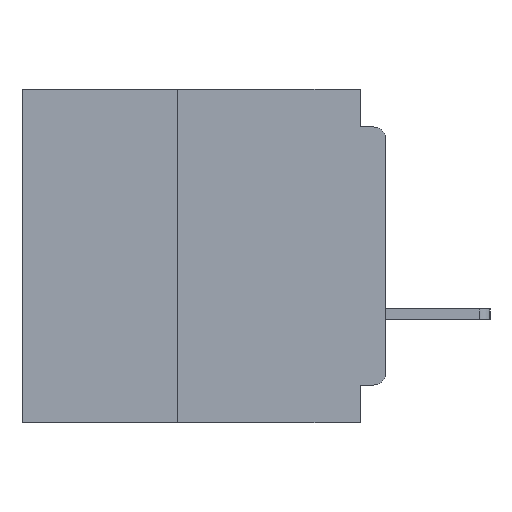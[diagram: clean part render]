
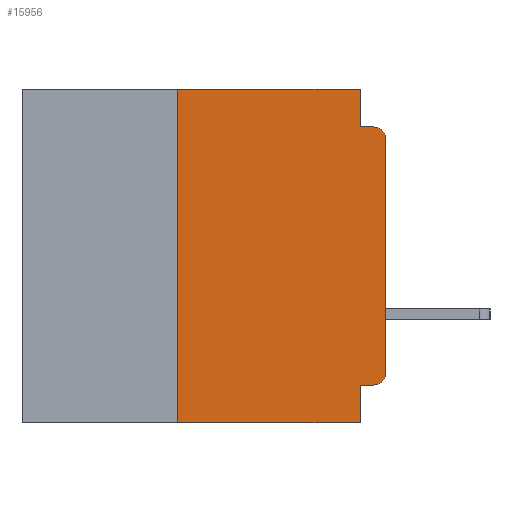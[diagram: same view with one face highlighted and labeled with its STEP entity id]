
A CAD part, left-side view. The second image highlights one B-rep face of the part: STEP entity #15956.
In plain terms, the highlighted planar face has unit normal (-1, 0, 0).
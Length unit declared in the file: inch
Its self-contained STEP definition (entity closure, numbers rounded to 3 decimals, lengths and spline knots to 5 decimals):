
#1579 = CARTESIAN_POINT ( 'NONE',  ( 0., 0.437, -0.4 ) ) ;
#1644 = DIRECTION ( 'NONE',  ( 0., 0., -1. ) ) ;
#3297 = VERTEX_POINT ( 'NONE', #16505 ) ;
#3374 = DIRECTION ( 'NONE',  ( -1., 0., 0. ) ) ;
#5253 = EDGE_CURVE ( 'NONE', #7783, #30090, #43500, .T. ) ;
#5803 = VERTEX_POINT ( 'NONE', #9554 ) ;
#6640 = DIRECTION ( 'NONE',  ( 0., 0., 1. ) ) ;
#7783 = VERTEX_POINT ( 'NONE', #48937 ) ;
#8978 = VERTEX_POINT ( 'NONE', #28548 ) ;
#9554 = CARTESIAN_POINT ( 'NONE',  ( 0., 0.031, -0.4 ) ) ;
#9669 = VECTOR ( 'NONE', #21164, 39.37008 ) ;
#9750 = CARTESIAN_POINT ( 'NONE',  ( 0., 0.015, -0.34 ) ) ;
#10940 = CARTESIAN_POINT ( 'NONE',  ( 0., 0.25, -0.4 ) ) ;
#11114 = LINE ( 'NONE', #27116, #21167 ) ;
#12034 = CARTESIAN_POINT ( 'NONE',  ( 0., 0., 0. ) ) ;
#12304 = VECTOR ( 'NONE', #52144, 39.37008 ) ;
#12464 = ORIENTED_EDGE ( 'NONE', *, *, #52574, .F. ) ;
#12562 = CARTESIAN_POINT ( 'NONE',  ( 0., 0., -0.355 ) ) ;
#12618 = CARTESIAN_POINT ( 'NONE',  ( 0., 0.25, -0.4 ) ) ;
#13251 = EDGE_CURVE ( 'NONE', #3297, #23100, #19534, .T. ) ;
#14091 = DIRECTION ( 'NONE',  ( 0., 0., -1. ) ) ;
#14128 = VECTOR ( 'NONE', #29550, 39.37008 ) ;
#15361 = ORIENTED_EDGE ( 'NONE', *, *, #41898, .T. ) ;
#15956 = ADVANCED_FACE ( 'NONE', ( #37205 ), #22993, .F. ) ;
#15974 = DIRECTION ( 'NONE',  ( 0., 0., 1. ) ) ;
#16505 = CARTESIAN_POINT ( 'NONE',  ( 0., 0.25, 0. ) ) ;
#16544 = ORIENTED_EDGE ( 'NONE', *, *, #5253, .F. ) ;
#16617 = VERTEX_POINT ( 'NONE', #44299 ) ;
#18028 = EDGE_CURVE ( 'NONE', #16617, #44447, #32406, .T. ) ;
#18341 = ORIENTED_EDGE ( 'NONE', *, *, #38912, .T. ) ;
#19534 = LINE ( 'NONE', #46771, #42001 ) ;
#20184 = CARTESIAN_POINT ( 'NONE',  ( 0., 0.015, -0.045 ) ) ;
#20460 = ORIENTED_EDGE ( 'NONE', *, *, #18028, .T. ) ;
#21164 = DIRECTION ( 'NONE',  ( 0., 1., 0. ) ) ;
#21167 = VECTOR ( 'NONE', #31429, 39.37008 ) ;
#22165 = EDGE_CURVE ( 'NONE', #23100, #8978, #11114, .T. ) ;
#22993 = PLANE ( 'NONE',  #26271 ) ;
#23100 = VERTEX_POINT ( 'NONE', #36058 ) ;
#23667 = LINE ( 'NONE', #39546, #12304 ) ;
#25241 = CARTESIAN_POINT ( 'NONE',  ( 0., 0., -0.045 ) ) ;
#25264 = ORIENTED_EDGE ( 'NONE', *, *, #22165, .F. ) ;
#25638 = CIRCLE ( 'NONE', #49632, 0.015 ) ;
#25844 = DIRECTION ( 'NONE',  ( 0., -1., 0. ) ) ;
#26271 = AXIS2_PLACEMENT_3D ( 'NONE', #52357, #27292, #1644 ) ;
#26833 = ORIENTED_EDGE ( 'NONE', *, *, #13251, .F. ) ;
#27116 = CARTESIAN_POINT ( 'NONE',  ( 0., 0.031, 0. ) ) ;
#27292 = DIRECTION ( 'NONE',  ( 1., 0., 0. ) ) ;
#28365 = CARTESIAN_POINT ( 'NONE',  ( 0., 0.031, -0.355 ) ) ;
#28548 = CARTESIAN_POINT ( 'NONE',  ( 0., 0.031, -0.045 ) ) ;
#29007 = CARTESIAN_POINT ( 'NONE',  ( 0., 0.015, -0.06 ) ) ;
#29541 = LINE ( 'NONE', #25241, #14128 ) ;
#29550 = DIRECTION ( 'NONE',  ( 0., -1., 0. ) ) ;
#30090 = VERTEX_POINT ( 'NONE', #28365 ) ;
#31429 = DIRECTION ( 'NONE',  ( 0., 0., -1. ) ) ;
#32406 = CIRCLE ( 'NONE', #41478, 0.015 ) ;
#33193 = ORIENTED_EDGE ( 'NONE', *, *, #40878, .T. ) ;
#33266 = DIRECTION ( 'NONE',  ( 0., 0., -1. ) ) ;
#33924 = VECTOR ( 'NONE', #35680, 39.37008 ) ;
#34425 = EDGE_CURVE ( 'NONE', #8978, #44447, #29541, .T. ) ;
#35285 = EDGE_LOOP ( 'NONE', ( #33193, #20460, #38125, #25264, #26833, #12464, #15361, #45844, #16544, #18341 ) ) ;
#35515 = VERTEX_POINT ( 'NONE', #12618 ) ;
#35680 = DIRECTION ( 'NONE',  ( 0., -1., 0. ) ) ;
#36058 = CARTESIAN_POINT ( 'NONE',  ( 0., 0.031, 0. ) ) ;
#37205 = FACE_OUTER_BOUND ( 'NONE', #35285, .T. ) ;
#38125 = ORIENTED_EDGE ( 'NONE', *, *, #34425, .F. ) ;
#38912 = EDGE_CURVE ( 'NONE', #7783, #54745, #25638, .T. ) ;
#39437 = DIRECTION ( 'NONE',  ( -1., 0., 0. ) ) ;
#39546 = CARTESIAN_POINT ( 'NONE',  ( 0., 0.031, -0.4 ) ) ;
#40878 = EDGE_CURVE ( 'NONE', #54745, #16617, #54219, .T. ) ;
#41478 = AXIS2_PLACEMENT_3D ( 'NONE', #29007, #3374, #33266 ) ;
#41573 = VECTOR ( 'NONE', #6640, 39.37008 ) ;
#41898 = EDGE_CURVE ( 'NONE', #35515, #5803, #45000, .T. ) ;
#42001 = VECTOR ( 'NONE', #25844, 39.37008 ) ;
#43500 = LINE ( 'NONE', #12562, #9669 ) ;
#44299 = CARTESIAN_POINT ( 'NONE',  ( 0., 0., -0.06 ) ) ;
#44447 = VERTEX_POINT ( 'NONE', #20184 ) ;
#44469 = VECTOR ( 'NONE', #15974, 39.37008 ) ;
#45000 = LINE ( 'NONE', #1579, #33924 ) ;
#45844 = ORIENTED_EDGE ( 'NONE', *, *, #53527, .F. ) ;
#46771 = CARTESIAN_POINT ( 'NONE',  ( 0., 0.437, 0. ) ) ;
#48225 = CARTESIAN_POINT ( 'NONE',  ( 0., 0., -0.34 ) ) ;
#48937 = CARTESIAN_POINT ( 'NONE',  ( 0., 0.015, -0.355 ) ) ;
#49632 = AXIS2_PLACEMENT_3D ( 'NONE', #9750, #39437, #14091 ) ;
#52144 = DIRECTION ( 'NONE',  ( 0., 0., -1. ) ) ;
#52357 = CARTESIAN_POINT ( 'NONE',  ( 0., 0.437, 0. ) ) ;
#52574 = EDGE_CURVE ( 'NONE', #35515, #3297, #52647, .T. ) ;
#52647 = LINE ( 'NONE', #10940, #41573 ) ;
#53527 = EDGE_CURVE ( 'NONE', #30090, #5803, #23667, .T. ) ;
#54219 = LINE ( 'NONE', #12034, #44469 ) ;
#54745 = VERTEX_POINT ( 'NONE', #48225 ) ;
